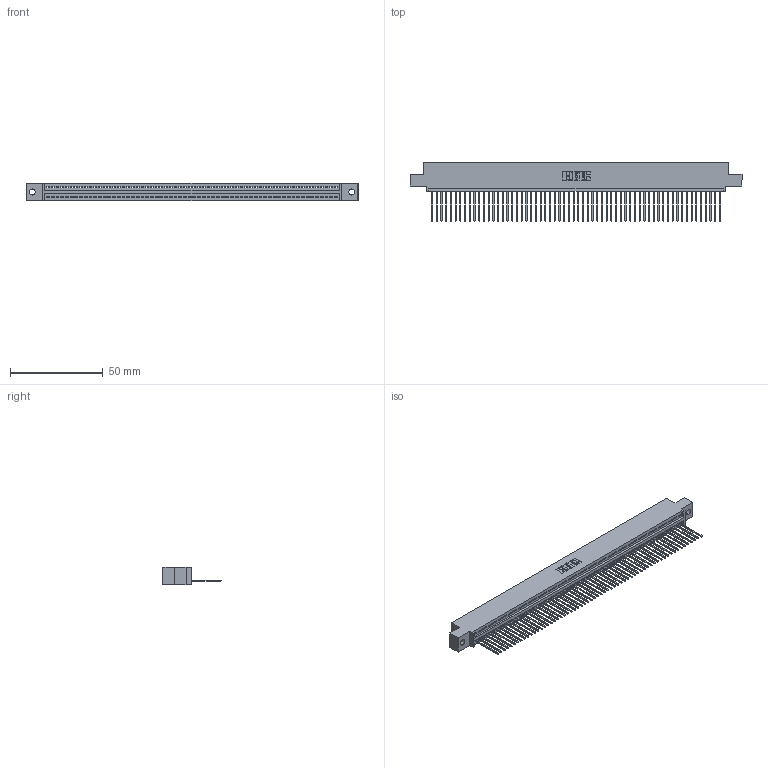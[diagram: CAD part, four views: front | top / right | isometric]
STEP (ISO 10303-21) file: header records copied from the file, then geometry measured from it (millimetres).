
FILE_DESCRIPTION (( 'STEP AP203' ), '1' );
FILE_NAME ('395-062-542-402.STEP', '2018-11-24T03:41:15', ( '' ), ( '' ), 'SwSTEP 2.0', 'SolidWorks 2016', '' );
FILE_SCHEMA (( 'CONFIG_CONTROL_DESIGN' ));
Length unit declared in the file: inch
Products named in the file (3): 345-292-001_345-293-142; 395-062-542-402; 345 Part_0.110 Offset - 0.128 Dia
Assembly tree (63 placements, depth 2):
  395-062-542-402
    345 Part_0.110 Offset - 0.128 Dia
    345-292-001_345-293-142  x62
Bounding box: 178.69 x 31.29 x 9.4 mm (x, y, z)
Volume: 17163.8 mm3; surface area: 23763.7 mm2
Topology: 63 solids, 63 shells, 3726 faces, 11265 edges, 7426 vertices
Faces by surface type: plane 2564, cylinder 1162
Entity records: 44123 total; most frequent: CARTESIAN_POINT 7650, ORIENTED_EDGE 7646, DIRECTION 6651, EDGE_CURVE 3823, LINE 3443, VECTOR 3443, VERTEX_POINT 2546, AXIS2_PLACEMENT_3D 1604
